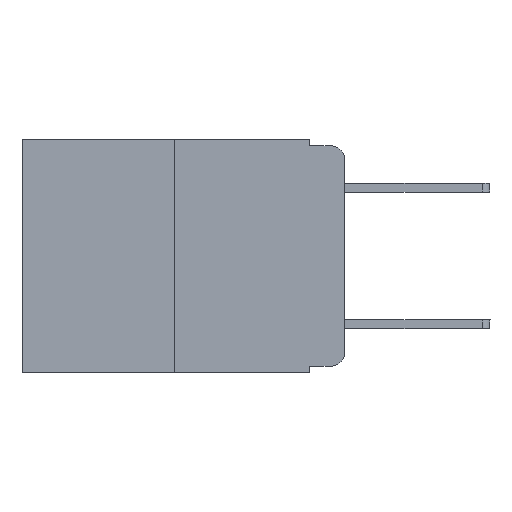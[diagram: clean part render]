
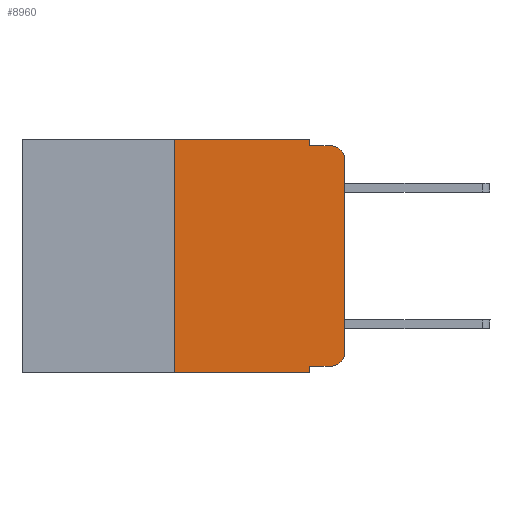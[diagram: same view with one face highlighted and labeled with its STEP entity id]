
A CAD part, left-side view. The second image highlights one B-rep face of the part: STEP entity #8960.
In plain terms, the highlighted planar face has unit normal (-1, 0, 0).
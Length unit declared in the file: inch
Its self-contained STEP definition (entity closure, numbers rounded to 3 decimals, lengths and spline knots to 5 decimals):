
#83 = EDGE_CURVE ( 'NONE', #9631, #10695, #13689, .T. ) ;
#258 = CARTESIAN_POINT ( 'NONE',  ( 0., 0.25, -0.343 ) ) ;
#318 = EDGE_LOOP ( 'NONE', ( #6485, #9871, #2027, #8447, #14184, #11918, #12235, #13072, #11982, #8448 ) ) ;
#355 = DIRECTION ( 'NONE',  ( 0., 0., -1. ) ) ;
#377 = EDGE_CURVE ( 'NONE', #2529, #564, #7745, .T. ) ;
#564 = VERTEX_POINT ( 'NONE', #6898 ) ;
#635 = VECTOR ( 'NONE', #972, 39.37008 ) ;
#758 = VECTOR ( 'NONE', #14378, 39.37008 ) ;
#820 = CARTESIAN_POINT ( 'NONE',  ( 0., 0.051, 0. ) ) ;
#889 = CARTESIAN_POINT ( 'NONE',  ( 0., 0.051, -0.333 ) ) ;
#972 = DIRECTION ( 'NONE',  ( 0., 0., 1. ) ) ;
#1241 = CARTESIAN_POINT ( 'NONE',  ( 0., 0., -0.03 ) ) ;
#1304 = VERTEX_POINT ( 'NONE', #10008 ) ;
#1434 = LINE ( 'NONE', #2840, #758 ) ;
#1436 = CARTESIAN_POINT ( 'NONE',  ( 0., 0., -0.313 ) ) ;
#1442 = VECTOR ( 'NONE', #4202, 39.37008 ) ;
#1528 = AXIS2_PLACEMENT_3D ( 'NONE', #8883, #7663, #13580 ) ;
#2027 = ORIENTED_EDGE ( 'NONE', *, *, #377, .F. ) ;
#2088 = PLANE ( 'NONE',  #1528 ) ;
#2276 = AXIS2_PLACEMENT_3D ( 'NONE', #2549, #14335, #12024 ) ;
#2529 = VERTEX_POINT ( 'NONE', #10779 ) ;
#2549 = CARTESIAN_POINT ( 'NONE',  ( 0., 0.02, -0.03 ) ) ;
#2840 = CARTESIAN_POINT ( 'NONE',  ( 0., 0.051, 0. ) ) ;
#2957 = EDGE_CURVE ( 'NONE', #5672, #2529, #1434, .T. ) ;
#3096 = VERTEX_POINT ( 'NONE', #889 ) ;
#3668 = EDGE_CURVE ( 'NONE', #10695, #564, #9585, .T. ) ;
#4063 = EDGE_CURVE ( 'NONE', #14126, #9631, #13086, .T. ) ;
#4105 = EDGE_CURVE ( 'NONE', #3096, #14126, #5326, .T. ) ;
#4202 = DIRECTION ( 'NONE',  ( 0., 0., 1. ) ) ;
#4292 = DIRECTION ( 'NONE',  ( 0., 0., -1. ) ) ;
#4478 = CARTESIAN_POINT ( 'NONE',  ( 0., 0.051, -0.01 ) ) ;
#5037 = CARTESIAN_POINT ( 'NONE',  ( 0., 0.051, -0.333 ) ) ;
#5120 = CARTESIAN_POINT ( 'NONE',  ( 0., 0.25, 0. ) ) ;
#5326 = LINE ( 'NONE', #5037, #7706 ) ;
#5548 = DIRECTION ( 'NONE',  ( 0., -1., 0. ) ) ;
#5672 = VERTEX_POINT ( 'NONE', #13886 ) ;
#6361 = EDGE_CURVE ( 'NONE', #3096, #1304, #8842, .T. ) ;
#6430 = CARTESIAN_POINT ( 'NONE',  ( 0., 0.473, -0.343 ) ) ;
#6453 = FACE_OUTER_BOUND ( 'NONE', #318, .T. ) ;
#6485 = ORIENTED_EDGE ( 'NONE', *, *, #83, .T. ) ;
#6617 = CARTESIAN_POINT ( 'NONE',  ( 0., 0.473, 0. ) ) ;
#6898 = CARTESIAN_POINT ( 'NONE',  ( 0., 0.02, -0.01 ) ) ;
#7214 = CARTESIAN_POINT ( 'NONE',  ( 0., 0., 0. ) ) ;
#7663 = DIRECTION ( 'NONE',  ( 1., 0., 0. ) ) ;
#7706 = VECTOR ( 'NONE', #14112, 39.37008 ) ;
#7745 = LINE ( 'NONE', #4478, #9407 ) ;
#7845 = VECTOR ( 'NONE', #8783, 39.37008 ) ;
#7983 = CARTESIAN_POINT ( 'NONE',  ( 0., 0.25, 0. ) ) ;
#8064 = EDGE_CURVE ( 'NONE', #10494, #1304, #14776, .T. ) ;
#8447 = ORIENTED_EDGE ( 'NONE', *, *, #2957, .F. ) ;
#8448 = ORIENTED_EDGE ( 'NONE', *, *, #4063, .T. ) ;
#8783 = DIRECTION ( 'NONE',  ( 0., -1., 0. ) ) ;
#8842 = LINE ( 'NONE', #820, #14670 ) ;
#8883 = CARTESIAN_POINT ( 'NONE',  ( 0., 0.473, 0. ) ) ;
#8889 = CARTESIAN_POINT ( 'NONE',  ( 0., 0.02, -0.333 ) ) ;
#8960 = ADVANCED_FACE ( 'NONE', ( #6453 ), #2088, .F. ) ;
#9386 = AXIS2_PLACEMENT_3D ( 'NONE', #12892, #9422, #355 ) ;
#9407 = VECTOR ( 'NONE', #5548, 39.37008 ) ;
#9422 = DIRECTION ( 'NONE',  ( -1., 0., 0. ) ) ;
#9585 = CIRCLE ( 'NONE', #2276, 0.02 ) ;
#9631 = VERTEX_POINT ( 'NONE', #1436 ) ;
#9871 = ORIENTED_EDGE ( 'NONE', *, *, #3668, .T. ) ;
#9930 = VERTEX_POINT ( 'NONE', #7983 ) ;
#10008 = CARTESIAN_POINT ( 'NONE',  ( 0., 0.051, -0.343 ) ) ;
#10101 = EDGE_CURVE ( 'NONE', #9930, #5672, #14812, .T. ) ;
#10494 = VERTEX_POINT ( 'NONE', #258 ) ;
#10695 = VERTEX_POINT ( 'NONE', #1241 ) ;
#10779 = CARTESIAN_POINT ( 'NONE',  ( 0., 0.051, -0.01 ) ) ;
#11136 = LINE ( 'NONE', #5120, #1442 ) ;
#11918 = ORIENTED_EDGE ( 'NONE', *, *, #13499, .F. ) ;
#11982 = ORIENTED_EDGE ( 'NONE', *, *, #4105, .T. ) ;
#12024 = DIRECTION ( 'NONE',  ( 0., 0., -1. ) ) ;
#12235 = ORIENTED_EDGE ( 'NONE', *, *, #8064, .T. ) ;
#12892 = CARTESIAN_POINT ( 'NONE',  ( 0., 0.02, -0.313 ) ) ;
#13072 = ORIENTED_EDGE ( 'NONE', *, *, #6361, .F. ) ;
#13086 = CIRCLE ( 'NONE', #9386, 0.02 ) ;
#13499 = EDGE_CURVE ( 'NONE', #10494, #9930, #11136, .T. ) ;
#13580 = DIRECTION ( 'NONE',  ( 0., 0., -1. ) ) ;
#13689 = LINE ( 'NONE', #7214, #635 ) ;
#13886 = CARTESIAN_POINT ( 'NONE',  ( 0., 0.051, 0. ) ) ;
#14112 = DIRECTION ( 'NONE',  ( 0., -1., 0. ) ) ;
#14126 = VERTEX_POINT ( 'NONE', #8889 ) ;
#14184 = ORIENTED_EDGE ( 'NONE', *, *, #10101, .F. ) ;
#14335 = DIRECTION ( 'NONE',  ( -1., 0., 0. ) ) ;
#14378 = DIRECTION ( 'NONE',  ( 0., 0., -1. ) ) ;
#14523 = DIRECTION ( 'NONE',  ( 0., -1., 0. ) ) ;
#14670 = VECTOR ( 'NONE', #4292, 39.37008 ) ;
#14754 = VECTOR ( 'NONE', #14523, 39.37008 ) ;
#14776 = LINE ( 'NONE', #6430, #7845 ) ;
#14812 = LINE ( 'NONE', #6617, #14754 ) ;
